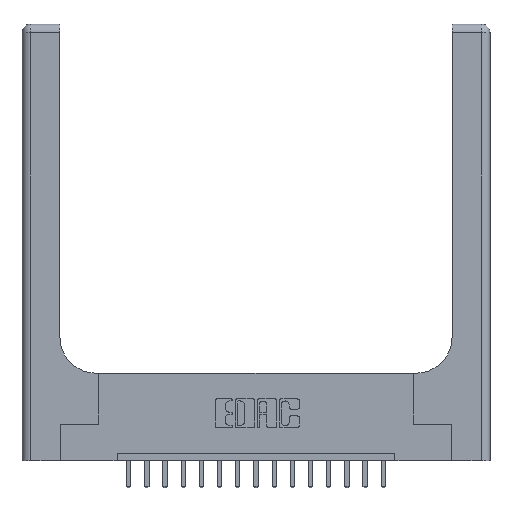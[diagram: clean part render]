
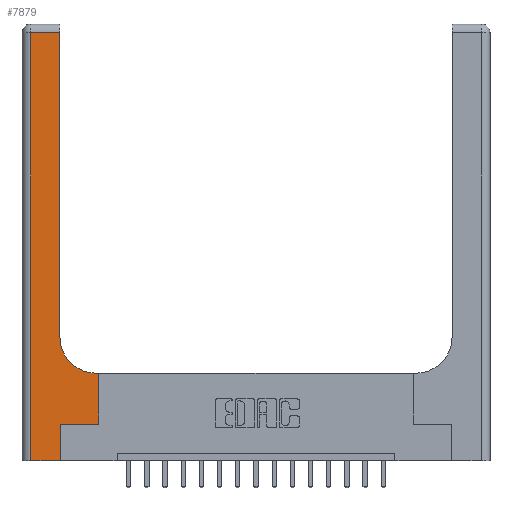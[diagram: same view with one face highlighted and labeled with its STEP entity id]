
A CAD part, top view. The second image highlights one B-rep face of the part: STEP entity #7879.
In plain terms, the highlighted planar face has unit normal (0, 0, 1).
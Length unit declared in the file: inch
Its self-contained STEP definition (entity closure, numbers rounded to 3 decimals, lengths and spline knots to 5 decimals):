
#224 = LINE ( 'NONE', #18000, #14334 ) ;
#552 = VERTEX_POINT ( 'NONE', #5675 ) ;
#721 = ORIENTED_EDGE ( 'NONE', *, *, #3979, .T. ) ;
#1370 = DIRECTION ( 'NONE',  ( 0., 1., 0. ) ) ;
#1395 = AXIS2_PLACEMENT_3D ( 'NONE', #11690, #14416, #4053 ) ;
#1406 = VERTEX_POINT ( 'NONE', #8805 ) ;
#1427 = CARTESIAN_POINT ( 'NONE',  ( 0.528, 0.25, 0.37 ) ) ;
#1570 = LINE ( 'NONE', #14644, #7544 ) ;
#1619 = CIRCLE ( 'NONE', #1395, 0.25 ) ;
#2280 = CARTESIAN_POINT ( 'NONE',  ( 0., 2.94, 0.37 ) ) ;
#2324 = VECTOR ( 'NONE', #12451, 39.37008 ) ;
#2661 = CARTESIAN_POINT ( 'NONE',  ( 0.528, 0.25, 0.37 ) ) ;
#2675 = VECTOR ( 'NONE', #5451, 39.37008 ) ;
#2879 = VECTOR ( 'NONE', #6914, 39.37008 ) ;
#3006 = CARTESIAN_POINT ( 'NONE',  ( 0.265, 0., 0.37 ) ) ;
#3628 = VECTOR ( 'NONE', #17814, 39.37008 ) ;
#3973 = VERTEX_POINT ( 'NONE', #5018 ) ;
#3979 = EDGE_CURVE ( 'NONE', #6531, #4995, #14936, .T. ) ;
#4038 = LINE ( 'NONE', #7116, #2675 ) ;
#4053 = DIRECTION ( 'NONE',  ( 1., 0., 0. ) ) ;
#4995 = VERTEX_POINT ( 'NONE', #3006 ) ;
#5018 = CARTESIAN_POINT ( 'NONE',  ( 0.26, 2.94, 0.37 ) ) ;
#5451 = DIRECTION ( 'NONE',  ( 1., 0., 0. ) ) ;
#5675 = CARTESIAN_POINT ( 'NONE',  ( 0.528, 0.6, 0.37 ) ) ;
#5921 = CARTESIAN_POINT ( 'NONE',  ( 0.06, 2.94, 0.37 ) ) ;
#6066 = ORIENTED_EDGE ( 'NONE', *, *, #9152, .T. ) ;
#6486 = CARTESIAN_POINT ( 'NONE',  ( 0.26, 0.6, 0.37 ) ) ;
#6531 = VERTEX_POINT ( 'NONE', #12895 ) ;
#6703 = LINE ( 'NONE', #2280, #3628 ) ;
#6750 = ORIENTED_EDGE ( 'NONE', *, *, #17694, .T. ) ;
#6914 = DIRECTION ( 'NONE',  ( 0., 1., 0. ) ) ;
#6918 = LINE ( 'NONE', #2661, #7578 ) ;
#7116 = CARTESIAN_POINT ( 'NONE',  ( 0.265, 0.25, 0.37 ) ) ;
#7126 = VERTEX_POINT ( 'NONE', #1427 ) ;
#7240 = EDGE_CURVE ( 'NONE', #552, #15888, #16155, .T. ) ;
#7353 = EDGE_CURVE ( 'NONE', #10360, #3973, #14598, .T. ) ;
#7544 = VECTOR ( 'NONE', #17474, 39.37008 ) ;
#7578 = VECTOR ( 'NONE', #1370, 39.37008 ) ;
#7781 = VECTOR ( 'NONE', #17749, 39.37008 ) ;
#7879 = ADVANCED_FACE ( 'NONE', ( #16692 ), #16653, .F. ) ;
#8205 = DIRECTION ( 'NONE',  ( 0., -1., 0. ) ) ;
#8440 = EDGE_CURVE ( 'NONE', #7126, #552, #6918, .T. ) ;
#8805 = CARTESIAN_POINT ( 'NONE',  ( 0.265, 0.25, 0.37 ) ) ;
#9123 = EDGE_LOOP ( 'NONE', ( #14890, #6750, #6066, #721, #16821, #10988, #12703, #10843, #16855 ) ) ;
#9152 = EDGE_CURVE ( 'NONE', #13544, #6531, #224, .T. ) ;
#10360 = VERTEX_POINT ( 'NONE', #16252 ) ;
#10843 = ORIENTED_EDGE ( 'NONE', *, *, #7240, .T. ) ;
#10988 = ORIENTED_EDGE ( 'NONE', *, *, #14232, .T. ) ;
#10997 = DIRECTION ( 'NONE',  ( 0., 0., -1. ) ) ;
#11690 = CARTESIAN_POINT ( 'NONE',  ( 0.51, 0.85, 0.37 ) ) ;
#11856 = AXIS2_PLACEMENT_3D ( 'NONE', #14022, #10997, #18128 ) ;
#12451 = DIRECTION ( 'NONE',  ( 1., 0., 0. ) ) ;
#12703 = ORIENTED_EDGE ( 'NONE', *, *, #8440, .T. ) ;
#12895 = CARTESIAN_POINT ( 'NONE',  ( 0.06, 0., 0.37 ) ) ;
#13544 = VERTEX_POINT ( 'NONE', #5921 ) ;
#13873 = CARTESIAN_POINT ( 'NONE',  ( 0.26, 3., 0.37 ) ) ;
#14022 = CARTESIAN_POINT ( 'NONE',  ( 0., 3., 0.37 ) ) ;
#14232 = EDGE_CURVE ( 'NONE', #1406, #7126, #4038, .T. ) ;
#14334 = VECTOR ( 'NONE', #8205, 39.37008 ) ;
#14344 = EDGE_CURVE ( 'NONE', #4995, #1406, #1570, .T. ) ;
#14416 = DIRECTION ( 'NONE',  ( 0., 0., -1. ) ) ;
#14598 = LINE ( 'NONE', #13873, #2879 ) ;
#14644 = CARTESIAN_POINT ( 'NONE',  ( 0.265, 0., 0.37 ) ) ;
#14662 = EDGE_CURVE ( 'NONE', #15888, #10360, #1619, .T. ) ;
#14890 = ORIENTED_EDGE ( 'NONE', *, *, #7353, .T. ) ;
#14936 = LINE ( 'NONE', #16281, #2324 ) ;
#15888 = VERTEX_POINT ( 'NONE', #16215 ) ;
#16155 = LINE ( 'NONE', #6486, #7781 ) ;
#16215 = CARTESIAN_POINT ( 'NONE',  ( 0.51, 0.6, 0.37 ) ) ;
#16252 = CARTESIAN_POINT ( 'NONE',  ( 0.26, 0.85, 0.37 ) ) ;
#16281 = CARTESIAN_POINT ( 'NONE',  ( 0., 0., 0.37 ) ) ;
#16653 = PLANE ( 'NONE',  #11856 ) ;
#16692 = FACE_OUTER_BOUND ( 'NONE', #9123, .T. ) ;
#16821 = ORIENTED_EDGE ( 'NONE', *, *, #14344, .T. ) ;
#16855 = ORIENTED_EDGE ( 'NONE', *, *, #14662, .T. ) ;
#17474 = DIRECTION ( 'NONE',  ( 0., 1., 0. ) ) ;
#17694 = EDGE_CURVE ( 'NONE', #3973, #13544, #6703, .T. ) ;
#17749 = DIRECTION ( 'NONE',  ( -1., 0., 0. ) ) ;
#17814 = DIRECTION ( 'NONE',  ( -1., 0., 0. ) ) ;
#18000 = CARTESIAN_POINT ( 'NONE',  ( 0.06, 3., 0.37 ) ) ;
#18128 = DIRECTION ( 'NONE',  ( -1., 0., 0. ) ) ;
